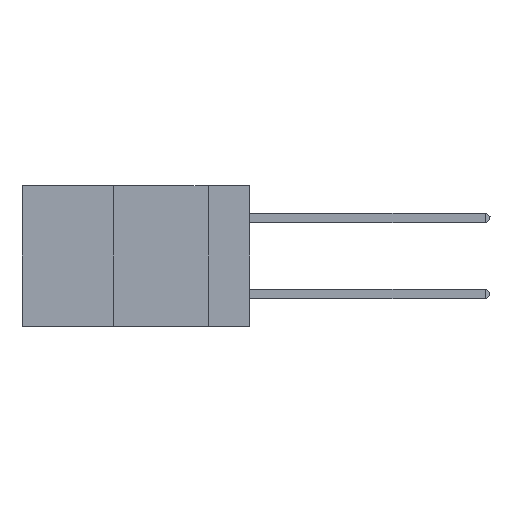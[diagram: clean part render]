
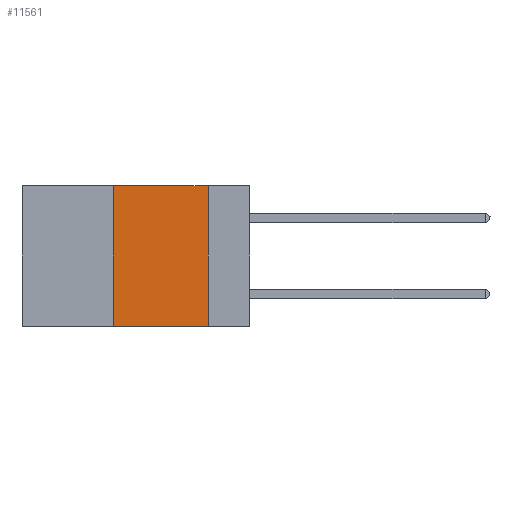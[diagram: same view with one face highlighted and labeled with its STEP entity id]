
A CAD part, left-side view. The second image highlights one B-rep face of the part: STEP entity #11561.
In plain terms, the highlighted planar face has unit normal (-1, 0, 0).
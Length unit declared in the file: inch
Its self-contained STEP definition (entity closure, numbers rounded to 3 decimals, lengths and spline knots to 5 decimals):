
#225 = EDGE_CURVE ( 'NONE', #37077, #22191, #31801, .T. ) ;
#497 = LINE ( 'NONE', #10432, #27069 ) ;
#856 = FACE_OUTER_BOUND ( 'NONE', #17818, .T. ) ;
#901 = CARTESIAN_POINT ( 'NONE',  ( 0., 0.36, 0. ) ) ;
#4962 = DIRECTION ( 'NONE',  ( 0., 0., 1. ) ) ;
#7117 = DIRECTION ( 'NONE',  ( 0., -1., 0. ) ) ;
#7766 = EDGE_CURVE ( 'NONE', #18023, #44111, #497, .T. ) ;
#10432 = CARTESIAN_POINT ( 'NONE',  ( 0., 0.6, 0. ) ) ;
#11561 = ADVANCED_FACE ( 'NONE', ( #856 ), #38551, .F. ) ;
#12315 = ORIENTED_EDGE ( 'NONE', *, *, #32720, .F. ) ;
#12778 = DIRECTION ( 'NONE',  ( 0., 0., -1. ) ) ;
#13190 = ORIENTED_EDGE ( 'NONE', *, *, #44232, .F. ) ;
#14400 = DIRECTION ( 'NONE',  ( 1., 0., 0. ) ) ;
#17818 = EDGE_LOOP ( 'NONE', ( #13190, #25698, #12315, #28981 ) ) ;
#18023 = VERTEX_POINT ( 'NONE', #41875 ) ;
#19331 = CARTESIAN_POINT ( 'NONE',  ( 0., 0.11, 0. ) ) ;
#22191 = VERTEX_POINT ( 'NONE', #28894 ) ;
#23383 = CARTESIAN_POINT ( 'NONE',  ( 0., 0.11, 0. ) ) ;
#25014 = CARTESIAN_POINT ( 'NONE',  ( 0., 0.6, 0. ) ) ;
#25698 = ORIENTED_EDGE ( 'NONE', *, *, #7766, .F. ) ;
#26560 = LINE ( 'NONE', #23383, #30879 ) ;
#27069 = VECTOR ( 'NONE', #28268, 39.37008 ) ;
#27303 = CARTESIAN_POINT ( 'NONE',  ( 0., 0.6, -0.37 ) ) ;
#28268 = DIRECTION ( 'NONE',  ( 0., -1., 0. ) ) ;
#28894 = CARTESIAN_POINT ( 'NONE',  ( 0., 0.11, -0.37 ) ) ;
#28981 = ORIENTED_EDGE ( 'NONE', *, *, #225, .T. ) ;
#30879 = VECTOR ( 'NONE', #12778, 39.37008 ) ;
#30904 = AXIS2_PLACEMENT_3D ( 'NONE', #25014, #14400, #35172 ) ;
#31801 = LINE ( 'NONE', #27303, #35619 ) ;
#32720 = EDGE_CURVE ( 'NONE', #37077, #18023, #35219, .T. ) ;
#33518 = CARTESIAN_POINT ( 'NONE',  ( 0., 0.36, -0.37 ) ) ;
#33813 = VECTOR ( 'NONE', #4962, 39.37008 ) ;
#35172 = DIRECTION ( 'NONE',  ( 0., 0., -1. ) ) ;
#35219 = LINE ( 'NONE', #901, #33813 ) ;
#35619 = VECTOR ( 'NONE', #7117, 39.37008 ) ;
#37077 = VERTEX_POINT ( 'NONE', #33518 ) ;
#38551 = PLANE ( 'NONE',  #30904 ) ;
#41875 = CARTESIAN_POINT ( 'NONE',  ( 0., 0.36, 0. ) ) ;
#44111 = VERTEX_POINT ( 'NONE', #19331 ) ;
#44232 = EDGE_CURVE ( 'NONE', #44111, #22191, #26560, .T. ) ;
